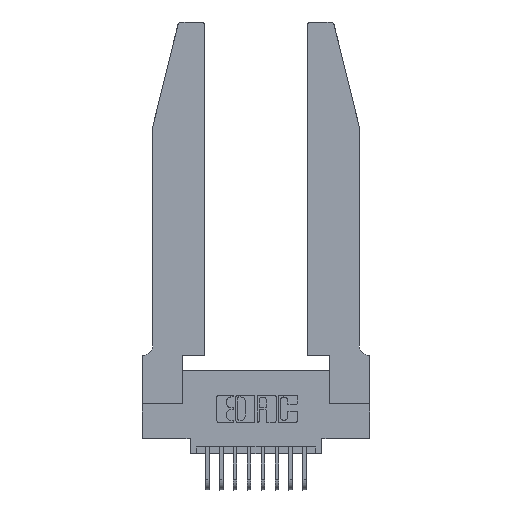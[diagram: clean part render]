
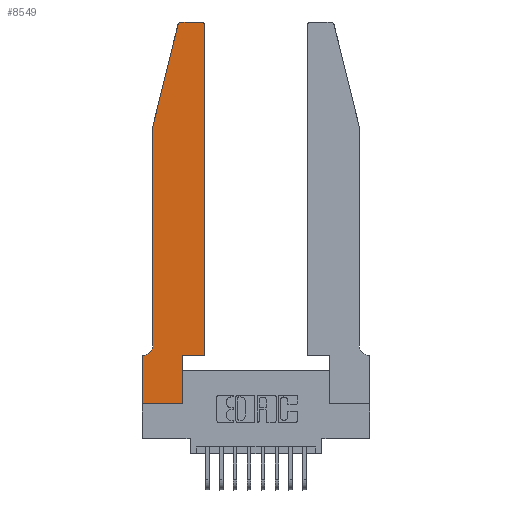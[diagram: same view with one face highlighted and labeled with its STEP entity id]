
A CAD part, top view. The second image highlights one B-rep face of the part: STEP entity #8549.
In plain terms, the highlighted planar face has unit normal (0, 0, 1).
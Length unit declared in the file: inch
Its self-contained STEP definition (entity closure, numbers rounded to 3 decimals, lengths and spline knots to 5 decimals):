
#95 = VECTOR ( 'NONE', #4927, 39.37008 ) ;
#204 = CARTESIAN_POINT ( 'NONE',  ( 0.284, 2.72, 0.37 ) ) ;
#384 = ORIENTED_EDGE ( 'NONE', *, *, #9746, .T. ) ;
#481 = ORIENTED_EDGE ( 'NONE', *, *, #6028, .T. ) ;
#576 = LINE ( 'NONE', #12989, #95 ) ;
#744 = VECTOR ( 'NONE', #5353, 39.37008 ) ;
#1364 = DIRECTION ( 'NONE',  ( 1., 0., 0. ) ) ;
#1655 = VERTEX_POINT ( 'NONE', #10924 ) ;
#1688 = DIRECTION ( 'NONE',  ( 0., 0., 1. ) ) ;
#1696 = EDGE_CURVE ( 'NONE', #12807, #6332, #8127, .T. ) ;
#1809 = CARTESIAN_POINT ( 'NONE',  ( 0., 0.35, 0.37 ) ) ;
#1951 = ORIENTED_EDGE ( 'NONE', *, *, #10163, .T. ) ;
#2139 = VERTEX_POINT ( 'NONE', #17421 ) ;
#2233 = ORIENTED_EDGE ( 'NONE', *, *, #15245, .T. ) ;
#2283 = VERTEX_POINT ( 'NONE', #8128 ) ;
#2446 = EDGE_CURVE ( 'NONE', #4693, #12807, #14485, .T. ) ;
#2691 = DIRECTION ( 'NONE',  ( 0., 0., -1. ) ) ;
#2805 = AXIS2_PLACEMENT_3D ( 'NONE', #10893, #2691, #12205 ) ;
#3123 = VERTEX_POINT ( 'NONE', #12411 ) ;
#3681 = EDGE_LOOP ( 'NONE', ( #481, #7616, #15802, #14377, #14721, #7435, #5129, #1951, #10897, #384, #2233, #9701 ) ) ;
#3837 = CARTESIAN_POINT ( 'NONE',  ( 0.4505, 0.35, 0.37 ) ) ;
#3949 = CARTESIAN_POINT ( 'NONE',  ( 0., 0., 0.37 ) ) ;
#4209 = AXIS2_PLACEMENT_3D ( 'NONE', #1809, #7367, #16537 ) ;
#4314 = DIRECTION ( 'NONE',  ( -1., 0., 0. ) ) ;
#4693 = VERTEX_POINT ( 'NONE', #8035 ) ;
#4927 = DIRECTION ( 'NONE',  ( 1., 0., 0. ) ) ;
#5129 = ORIENTED_EDGE ( 'NONE', *, *, #8279, .T. ) ;
#5353 = DIRECTION ( 'NONE',  ( -0.239, -0.971, 0. ) ) ;
#5637 = CARTESIAN_POINT ( 'NONE',  ( 0.0755, 2., 0.37 ) ) ;
#5859 = LINE ( 'NONE', #3949, #8670 ) ;
#5903 = VERTEX_POINT ( 'NONE', #10850 ) ;
#6028 = EDGE_CURVE ( 'NONE', #5903, #4693, #8970, .T. ) ;
#6056 = CARTESIAN_POINT ( 'NONE',  ( 0.0755, 0.35, 0.37 ) ) ;
#6332 = VERTEX_POINT ( 'NONE', #7561 ) ;
#6568 = LINE ( 'NONE', #6056, #13290 ) ;
#6657 = CARTESIAN_POINT ( 'NONE',  ( 0.2865, 0.35, 0.37 ) ) ;
#6685 = VERTEX_POINT ( 'NONE', #10943 ) ;
#6732 = VECTOR ( 'NONE', #12220, 39.37008 ) ;
#7367 = DIRECTION ( 'NONE',  ( 0., 0., 1. ) ) ;
#7435 = ORIENTED_EDGE ( 'NONE', *, *, #13811, .T. ) ;
#7561 = CARTESIAN_POINT ( 'NONE',  ( 0.0755, 2., 0.37 ) ) ;
#7606 = VERTEX_POINT ( 'NONE', #17072 ) ;
#7616 = ORIENTED_EDGE ( 'NONE', *, *, #2446, .T. ) ;
#7656 = EDGE_CURVE ( 'NONE', #6332, #2283, #11220, .T. ) ;
#8035 = CARTESIAN_POINT ( 'NONE',  ( 0.284, 2.75, 0.37 ) ) ;
#8127 = LINE ( 'NONE', #5637, #744 ) ;
#8128 = CARTESIAN_POINT ( 'NONE',  ( 0.0755, 0.42, 0.37 ) ) ;
#8222 = CARTESIAN_POINT ( 'NONE',  ( 0., 0., 0.37 ) ) ;
#8224 = VECTOR ( 'NONE', #12098, 39.37008 ) ;
#8279 = EDGE_CURVE ( 'NONE', #2139, #12000, #5859, .T. ) ;
#8298 = EDGE_CURVE ( 'NONE', #1655, #6685, #11826, .T. ) ;
#8549 = ADVANCED_FACE ( 'NONE', ( #12402 ), #15261, .T. ) ;
#8670 = VECTOR ( 'NONE', #12039, 39.37008 ) ;
#8735 = VERTEX_POINT ( 'NONE', #12132 ) ;
#8893 = LINE ( 'NONE', #11960, #15412 ) ;
#8970 = LINE ( 'NONE', #9733, #12091 ) ;
#9701 = ORIENTED_EDGE ( 'NONE', *, *, #14379, .T. ) ;
#9733 = CARTESIAN_POINT ( 'NONE',  ( 0.2605, 2.75, 0.37 ) ) ;
#9746 = EDGE_CURVE ( 'NONE', #6685, #8735, #13779, .T. ) ;
#9837 = EDGE_CURVE ( 'NONE', #2283, #3123, #12982, .T. ) ;
#9895 = VECTOR ( 'NONE', #17049, 39.37008 ) ;
#9946 = CARTESIAN_POINT ( 'NONE',  ( 0.4205, 2.72, 0.37 ) ) ;
#10145 = DIRECTION ( 'NONE',  ( -1., 0., 0. ) ) ;
#10163 = EDGE_CURVE ( 'NONE', #12000, #1655, #576, .T. ) ;
#10850 = CARTESIAN_POINT ( 'NONE',  ( 0.4205, 2.75, 0.37 ) ) ;
#10893 = CARTESIAN_POINT ( 'NONE',  ( 0.0055, 0.42, 0.37 ) ) ;
#10897 = ORIENTED_EDGE ( 'NONE', *, *, #8298, .T. ) ;
#10924 = CARTESIAN_POINT ( 'NONE',  ( 0.2865, 0., 0.37 ) ) ;
#10943 = CARTESIAN_POINT ( 'NONE',  ( 0.2865, 0.35, 0.37 ) ) ;
#11220 = LINE ( 'NONE', #13529, #6732 ) ;
#11298 = DIRECTION ( 'NONE',  ( 1., 0., 0. ) ) ;
#11826 = LINE ( 'NONE', #6657, #8224 ) ;
#11960 = CARTESIAN_POINT ( 'NONE',  ( 0.4505, 0.35, 0.37 ) ) ;
#12000 = VERTEX_POINT ( 'NONE', #8222 ) ;
#12039 = DIRECTION ( 'NONE',  ( 0., -1., 0. ) ) ;
#12091 = VECTOR ( 'NONE', #4314, 39.37008 ) ;
#12098 = DIRECTION ( 'NONE',  ( 0., 1., 0. ) ) ;
#12132 = CARTESIAN_POINT ( 'NONE',  ( 0.4505, 0.35, 0.37 ) ) ;
#12205 = DIRECTION ( 'NONE',  ( -1., 0., 0. ) ) ;
#12220 = DIRECTION ( 'NONE',  ( 0., -1., 0. ) ) ;
#12402 = FACE_OUTER_BOUND ( 'NONE', #3681, .T. ) ;
#12411 = CARTESIAN_POINT ( 'NONE',  ( 0.0055, 0.35, 0.37 ) ) ;
#12807 = VERTEX_POINT ( 'NONE', #12987 ) ;
#12982 = CIRCLE ( 'NONE', #2805, 0.07 ) ;
#12987 = CARTESIAN_POINT ( 'NONE',  ( 0.25487, 2.72718, 0.37 ) ) ;
#12989 = CARTESIAN_POINT ( 'NONE',  ( 0., 0., 0.37 ) ) ;
#13250 = DIRECTION ( 'NONE',  ( 0., 1., 0. ) ) ;
#13290 = VECTOR ( 'NONE', #10145, 39.37008 ) ;
#13529 = CARTESIAN_POINT ( 'NONE',  ( 0.0755, 2., 0.37 ) ) ;
#13779 = LINE ( 'NONE', #3837, #9895 ) ;
#13811 = EDGE_CURVE ( 'NONE', #3123, #2139, #6568, .T. ) ;
#14309 = DIRECTION ( 'NONE',  ( 0., 0., 1. ) ) ;
#14377 = ORIENTED_EDGE ( 'NONE', *, *, #7656, .T. ) ;
#14379 = EDGE_CURVE ( 'NONE', #7606, #5903, #14633, .T. ) ;
#14485 = CIRCLE ( 'NONE', #16017, 0.03 ) ;
#14633 = CIRCLE ( 'NONE', #15161, 0.03 ) ;
#14721 = ORIENTED_EDGE ( 'NONE', *, *, #9837, .T. ) ;
#15161 = AXIS2_PLACEMENT_3D ( 'NONE', #9946, #1688, #11298 ) ;
#15245 = EDGE_CURVE ( 'NONE', #8735, #7606, #8893, .T. ) ;
#15261 = PLANE ( 'NONE',  #4209 ) ;
#15412 = VECTOR ( 'NONE', #13250, 39.37008 ) ;
#15802 = ORIENTED_EDGE ( 'NONE', *, *, #1696, .T. ) ;
#16017 = AXIS2_PLACEMENT_3D ( 'NONE', #204, #14309, #1364 ) ;
#16537 = DIRECTION ( 'NONE',  ( 1., 0., 0. ) ) ;
#17049 = DIRECTION ( 'NONE',  ( 1., 0., 0. ) ) ;
#17072 = CARTESIAN_POINT ( 'NONE',  ( 0.4505, 2.72, 0.37 ) ) ;
#17421 = CARTESIAN_POINT ( 'NONE',  ( 0., 0.35, 0.37 ) ) ;
